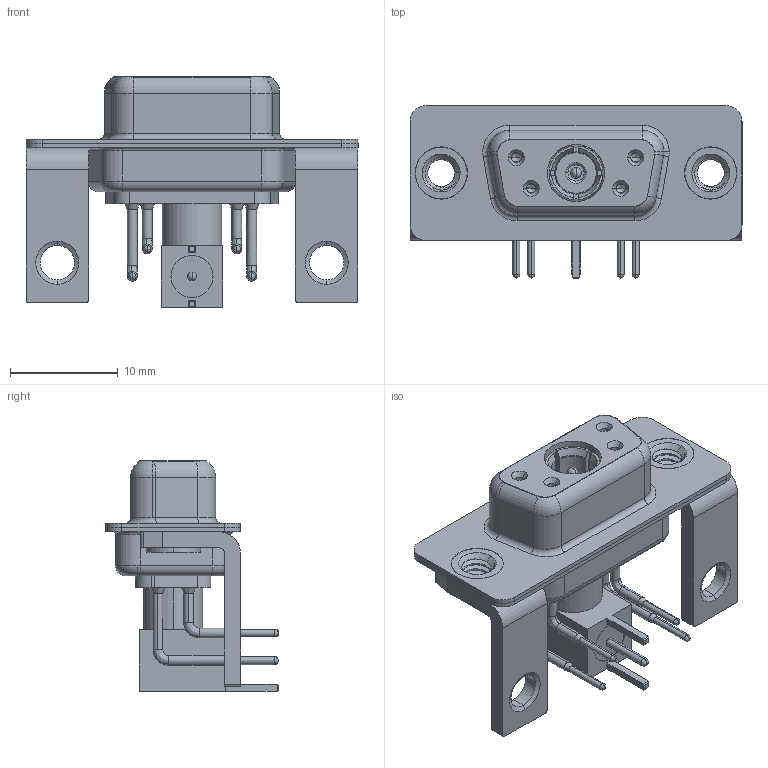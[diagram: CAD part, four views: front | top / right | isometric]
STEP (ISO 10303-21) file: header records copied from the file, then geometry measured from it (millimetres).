
FILE_DESCRIPTION (( 'STEP AP203' ), '1' );
FILE_NAME ('630-5W1-240-5NC.STEP', '2022-05-27T07:26:38', ( '' ), ( '' ), 'SwSTEP 2.0', 'SolidWorks 2020', '' );
FILE_SCHEMA (( 'CONFIG_CONTROL_DESIGN' ));
Length unit declared in the file: millimetre
Products named in the file (15): 630Combo Stabilizer Bracket; RA Back Shell; Locking Collar; Insulator Pin_Straight PC Tail; 630Combo Housing_5W1; 630-5W1-240-5NC; Pin_RA; 630Combo Threaded Rivet_B; 630Combo Contact Row 2; 630Combo Shell Rear_09 Contacts; Co-Ax Plug Assy_RA; 630Combo Contact Row 1; Insulator RA Pin; 630Combo Shell Front_09 Contacts; Co-Ax Plug_RA PC Tail
Assembly tree (18 placements, depth 3):
  630-5W1-240-5NC
    630Combo Housing_5W1
    630Combo Shell Front_09 Contacts
    630Combo Shell Rear_09 Contacts
    630Combo Threaded Rivet_B  x2
    630Combo Stabilizer Bracket  x2
    Co-Ax Plug Assy_RA
      Co-Ax Plug_RA PC Tail
      Insulator Pin_Straight PC Tail
      Pin_RA
      Locking Collar
      RA Back Shell
      Insulator RA Pin
    630Combo Contact Row 1  x2
    630Combo Contact Row 2  x2
Bounding box: 30.8 x 16 x 21.41 mm (x, y, z)
Volume: 2233.3 mm3; surface area: 5599.6 mm2
Topology: 17 solids, 17 shells, 697 faces, 1726 edges, 1084 vertices
Faces by surface type: cylinder 312, plane 214, cone 81, torus 63, bspline 23, sphere 4
Entity records: 20113 total; most frequent: CARTESIAN_POINT 4822, DIRECTION 3059, ORIENTED_EDGE 2722, EDGE_CURVE 1361, AXIS2_PLACEMENT_3D 1234, VERTEX_POINT 863, CIRCLE 659, EDGE_LOOP 642
